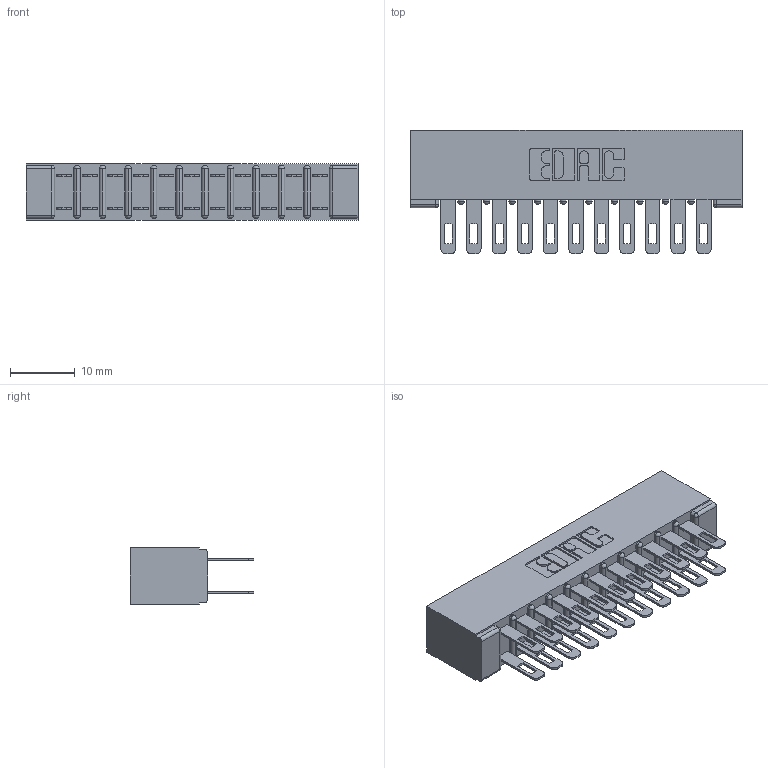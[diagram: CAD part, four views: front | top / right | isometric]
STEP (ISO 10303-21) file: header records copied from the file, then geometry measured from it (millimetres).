
FILE_DESCRIPTION (( 'STEP AP203' ), '1' );
FILE_NAME ('357-022-400-201.STEP', '2020-10-02T22:49:38', ( '' ), ( '' ), 'SwSTEP 2.0', 'SolidWorks 2020', '' );
FILE_SCHEMA (( 'CONFIG_CONTROL_DESIGN' ));
Length unit declared in the file: inch
Products named in the file (3): 307-290-001_500; 307 Part_No Mounting Lugs; 357-022-400-201
Assembly tree (23 placements, depth 2):
  357-022-400-201
    307 Part_No Mounting Lugs
    307-290-001_500  x22
Bounding box: 51.46 x 19.18 x 8.71 mm (x, y, z)
Volume: 3663.4 mm3; surface area: 6717.3 mm2
Topology: 23 solids, 23 shells, 1134 faces, 3159 edges, 2042 vertices
Faces by surface type: plane 726, cylinder 384, sphere 24
Entity records: 13300 total; most frequent: CARTESIAN_POINT 2179, ORIENTED_EDGE 2154, DIRECTION 2149, EDGE_CURVE 1077, LINE 813, VECTOR 813, VERTEX_POINT 698, AXIS2_PLACEMENT_3D 668
